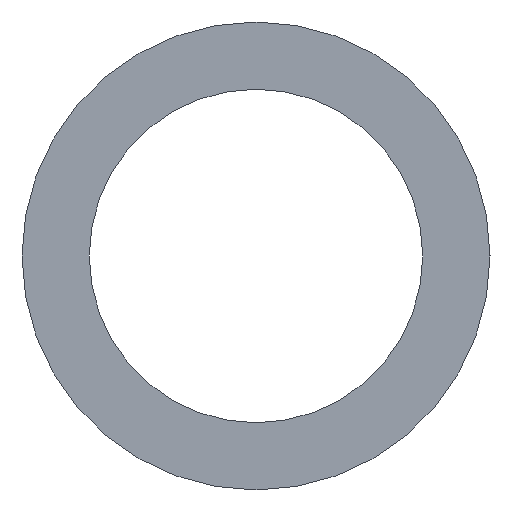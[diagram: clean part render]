
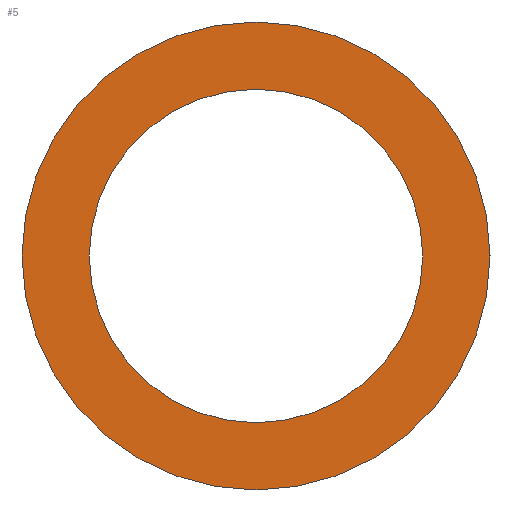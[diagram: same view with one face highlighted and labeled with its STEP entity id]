
A CAD part, left-side view. The second image highlights one B-rep face of the part: STEP entity #5.
In plain terms, the highlighted planar face has unit normal (-1, 0, 0).
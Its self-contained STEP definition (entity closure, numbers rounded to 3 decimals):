
#5 = ADVANCED_FACE ( 'NONE', ( #269, #261 ), #161, .F. ) ;
#23 = AXIS2_PLACEMENT_3D ( 'NONE', #138, #169, #170 ) ;
#26 = AXIS2_PLACEMENT_3D ( 'NONE', #141, #142, #166 ) ;
#50 = EDGE_CURVE ( 'NONE', #229, #191, #272, .T. ) ;
#53 = EDGE_CURVE ( 'NONE', #231, #242, #262, .T. ) ;
#59 = AXIS2_PLACEMENT_3D ( 'NONE', #122, #86, #135 ) ;
#60 = AXIS2_PLACEMENT_3D ( 'NONE', #163, #123, #117 ) ;
#62 = AXIS2_PLACEMENT_3D ( 'NONE', #131, #159, #160 ) ;
#69 = EDGE_CURVE ( 'NONE', #191, #229, #286, .T. ) ;
#78 = EDGE_CURVE ( 'NONE', #242, #231, #288, .T. ) ;
#86 = DIRECTION ( 'NONE',  ( 1., 0., 0. ) ) ;
#97 = CARTESIAN_POINT ( 'NONE',  ( 0., 0., -2.85 ) ) ;
#99 = CARTESIAN_POINT ( 'NONE',  ( 0., 0., 2.85 ) ) ;
#108 = CARTESIAN_POINT ( 'NONE',  ( 0., 0., -4. ) ) ;
#117 = DIRECTION ( 'NONE',  ( 0., 0., -1. ) ) ;
#122 = CARTESIAN_POINT ( 'NONE',  ( 0., 0., 0. ) ) ;
#123 = DIRECTION ( 'NONE',  ( 1., 0., 0. ) ) ;
#131 = CARTESIAN_POINT ( 'NONE',  ( 0., 0., 0. ) ) ;
#135 = DIRECTION ( 'NONE',  ( 0., 0., -1. ) ) ;
#138 = CARTESIAN_POINT ( 'NONE',  ( 0., 0., 0. ) ) ;
#141 = CARTESIAN_POINT ( 'NONE',  ( 0., 0., 0. ) ) ;
#142 = DIRECTION ( 'NONE',  ( 1., 0., 0. ) ) ;
#159 = DIRECTION ( 'NONE',  ( 1., 0., 0. ) ) ;
#160 = DIRECTION ( 'NONE',  ( 0., 0., -1. ) ) ;
#161 = PLANE ( 'NONE',  #60 ) ;
#163 = CARTESIAN_POINT ( 'NONE',  ( 0., 0., 0. ) ) ;
#166 = DIRECTION ( 'NONE',  ( 0., 0., -1. ) ) ;
#169 = DIRECTION ( 'NONE',  ( 1., 0., 0. ) ) ;
#170 = DIRECTION ( 'NONE',  ( 0., 0., -1. ) ) ;
#175 = CARTESIAN_POINT ( 'NONE',  ( 0., 0., 4. ) ) ;
#191 = VERTEX_POINT ( 'NONE', #175 ) ;
#199 = ORIENTED_EDGE ( 'NONE', *, *, #50, .F. ) ;
#200 = ORIENTED_EDGE ( 'NONE', *, *, #69, .F. ) ;
#201 = ORIENTED_EDGE ( 'NONE', *, *, #78, .T. ) ;
#204 = EDGE_LOOP ( 'NONE', ( #239, #201 ) ) ;
#207 = EDGE_LOOP ( 'NONE', ( #200, #199 ) ) ;
#229 = VERTEX_POINT ( 'NONE', #108 ) ;
#231 = VERTEX_POINT ( 'NONE', #97 ) ;
#239 = ORIENTED_EDGE ( 'NONE', *, *, #53, .T. ) ;
#242 = VERTEX_POINT ( 'NONE', #99 ) ;
#261 = FACE_OUTER_BOUND ( 'NONE', #207, .T. ) ;
#262 = CIRCLE ( 'NONE', #62, 2.85 ) ;
#269 = FACE_BOUND ( 'NONE', #204, .T. ) ;
#272 = CIRCLE ( 'NONE', #59, 4. ) ;
#286 = CIRCLE ( 'NONE', #26, 4. ) ;
#288 = CIRCLE ( 'NONE', #23, 2.85 ) ;
